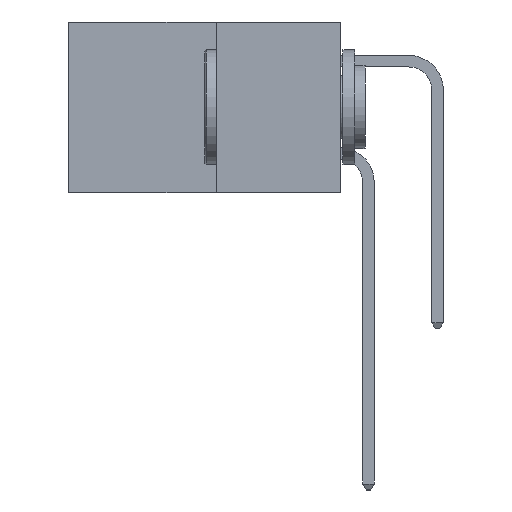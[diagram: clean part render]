
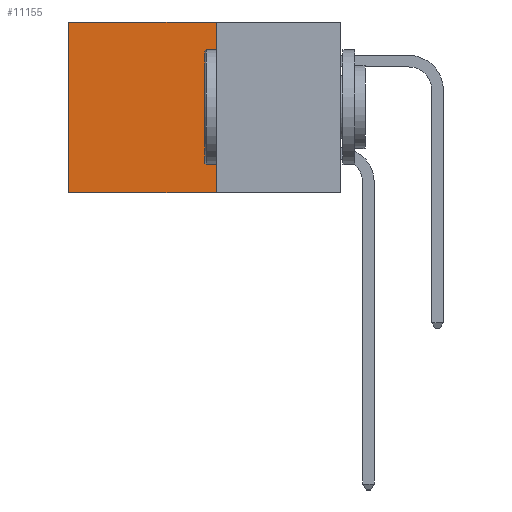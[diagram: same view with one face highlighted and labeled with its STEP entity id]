
A CAD part, left-side view. The second image highlights one B-rep face of the part: STEP entity #11155.
In plain terms, the highlighted planar face has unit normal (-1, 0, 0).
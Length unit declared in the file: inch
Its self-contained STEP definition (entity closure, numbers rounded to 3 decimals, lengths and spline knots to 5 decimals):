
#634 = DIRECTION ( 'NONE',  ( 1., 0., 0. ) ) ;
#1809 = DIRECTION ( 'NONE',  ( 0., 1., 0. ) ) ;
#1851 = DIRECTION ( 'NONE',  ( 0., 0., -1. ) ) ;
#2164 = VERTEX_POINT ( 'NONE', #28272 ) ;
#2166 = DIRECTION ( 'NONE',  ( 0., 1., 0. ) ) ;
#3538 = VERTEX_POINT ( 'NONE', #18677 ) ;
#4892 = VERTEX_POINT ( 'NONE', #22487 ) ;
#8009 = ORIENTED_EDGE ( 'NONE', *, *, #21035, .T. ) ;
#8891 = VECTOR ( 'NONE', #1851, 39.37008 ) ;
#9073 = AXIS2_PLACEMENT_3D ( 'NONE', #28778, #634, #17105 ) ;
#11155 = ADVANCED_FACE ( 'NONE', ( #18062 ), #21687, .F. ) ;
#11226 = CARTESIAN_POINT ( 'NONE',  ( 0.277, 0.59, -0.37 ) ) ;
#11535 = EDGE_LOOP ( 'NONE', ( #8009, #11537, #14996, #17816 ) ) ;
#11537 = ORIENTED_EDGE ( 'NONE', *, *, #28183, .F. ) ;
#11620 = EDGE_CURVE ( 'NONE', #2164, #3538, #20280, .T. ) ;
#12150 = VECTOR ( 'NONE', #23319, 39.37008 ) ;
#12276 = VECTOR ( 'NONE', #1809, 39.37008 ) ;
#14994 = VERTEX_POINT ( 'NONE', #21496 ) ;
#14996 = ORIENTED_EDGE ( 'NONE', *, *, #22723, .F. ) ;
#17105 = DIRECTION ( 'NONE',  ( 0., 0., -1. ) ) ;
#17816 = ORIENTED_EDGE ( 'NONE', *, *, #11620, .T. ) ;
#18062 = FACE_OUTER_BOUND ( 'NONE', #11535, .T. ) ;
#18593 = CARTESIAN_POINT ( 'NONE',  ( 0.277, 0.27, -0.37 ) ) ;
#18677 = CARTESIAN_POINT ( 'NONE',  ( 0.277, 0.59, 0. ) ) ;
#19231 = LINE ( 'NONE', #27564, #12276 ) ;
#20280 = LINE ( 'NONE', #30264, #25804 ) ;
#21035 = EDGE_CURVE ( 'NONE', #3538, #14994, #27604, .T. ) ;
#21496 = CARTESIAN_POINT ( 'NONE',  ( 0.277, 0.59, -0.37 ) ) ;
#21687 = PLANE ( 'NONE',  #9073 ) ;
#22487 = CARTESIAN_POINT ( 'NONE',  ( 0.277, 0.27, -0.37 ) ) ;
#22723 = EDGE_CURVE ( 'NONE', #2164, #4892, #24635, .T. ) ;
#23319 = DIRECTION ( 'NONE',  ( 0., 0., -1. ) ) ;
#24635 = LINE ( 'NONE', #18593, #12150 ) ;
#25804 = VECTOR ( 'NONE', #2166, 39.37008 ) ;
#27564 = CARTESIAN_POINT ( 'NONE',  ( 0.277, 0.27, -0.37 ) ) ;
#27604 = LINE ( 'NONE', #11226, #8891 ) ;
#28183 = EDGE_CURVE ( 'NONE', #4892, #14994, #19231, .T. ) ;
#28272 = CARTESIAN_POINT ( 'NONE',  ( 0.277, 0.27, 0. ) ) ;
#28778 = CARTESIAN_POINT ( 'NONE',  ( 0.277, 0.27, -0.37 ) ) ;
#30264 = CARTESIAN_POINT ( 'NONE',  ( 0.277, 0.27, 0. ) ) ;
